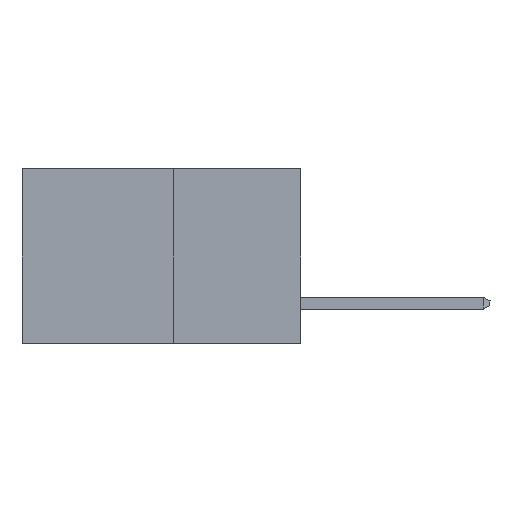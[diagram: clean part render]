
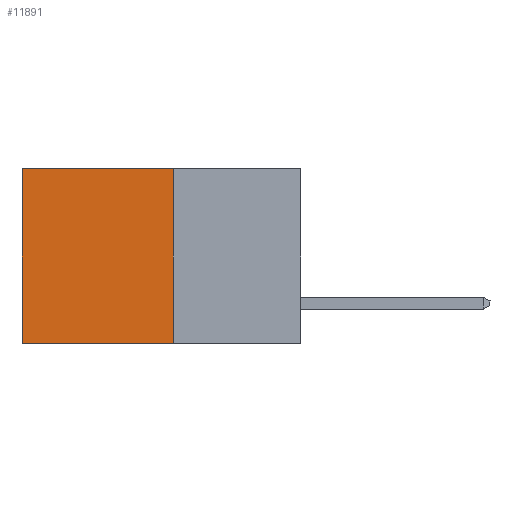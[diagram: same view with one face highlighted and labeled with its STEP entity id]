
A CAD part, left-side view. The second image highlights one B-rep face of the part: STEP entity #11891.
In plain terms, the highlighted planar face has unit normal (-1, 0, 0).
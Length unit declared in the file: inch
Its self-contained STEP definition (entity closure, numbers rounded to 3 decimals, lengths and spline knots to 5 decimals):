
#1458 = DIRECTION ( 'NONE',  ( 1., 0., 0. ) ) ;
#1577 = CARTESIAN_POINT ( 'NONE',  ( 0.277, 0.59, 0. ) ) ;
#1660 = VERTEX_POINT ( 'NONE', #1577 ) ;
#1937 = CARTESIAN_POINT ( 'NONE',  ( 0.277, 0.27, 0. ) ) ;
#2362 = DIRECTION ( 'NONE',  ( 0., 1., 0. ) ) ;
#2758 = LINE ( 'NONE', #12853, #5397 ) ;
#2946 = CARTESIAN_POINT ( 'NONE',  ( 0.277, 0.27, 0. ) ) ;
#2965 = DIRECTION ( 'NONE',  ( 0., 1., 0. ) ) ;
#3231 = VERTEX_POINT ( 'NONE', #8208 ) ;
#4039 = VERTEX_POINT ( 'NONE', #1937 ) ;
#4247 = ORIENTED_EDGE ( 'NONE', *, *, #6559, .T. ) ;
#4698 = EDGE_CURVE ( 'NONE', #4039, #1660, #4982, .T. ) ;
#4809 = VERTEX_POINT ( 'NONE', #12917 ) ;
#4841 = ORIENTED_EDGE ( 'NONE', *, *, #4698, .T. ) ;
#4982 = LINE ( 'NONE', #2946, #10055 ) ;
#5397 = VECTOR ( 'NONE', #9606, 39.37008 ) ;
#5882 = CARTESIAN_POINT ( 'NONE',  ( 0.277, 0.27, -0.37 ) ) ;
#6417 = CARTESIAN_POINT ( 'NONE',  ( 0.277, 0.27, -0.37 ) ) ;
#6559 = EDGE_CURVE ( 'NONE', #1660, #4809, #2758, .T. ) ;
#7026 = LINE ( 'NONE', #5882, #9393 ) ;
#7212 = ORIENTED_EDGE ( 'NONE', *, *, #7262, .F. ) ;
#7262 = EDGE_CURVE ( 'NONE', #4039, #3231, #12898, .T. ) ;
#7504 = ORIENTED_EDGE ( 'NONE', *, *, #12745, .F. ) ;
#7526 = CARTESIAN_POINT ( 'NONE',  ( 0.277, 0.27, -0.37 ) ) ;
#8208 = CARTESIAN_POINT ( 'NONE',  ( 0.277, 0.27, -0.37 ) ) ;
#8508 = DIRECTION ( 'NONE',  ( 0., 0., -1. ) ) ;
#9393 = VECTOR ( 'NONE', #2965, 39.37008 ) ;
#9435 = AXIS2_PLACEMENT_3D ( 'NONE', #7526, #1458, #8508 ) ;
#9606 = DIRECTION ( 'NONE',  ( 0., 0., -1. ) ) ;
#10055 = VECTOR ( 'NONE', #2362, 39.37008 ) ;
#10074 = DIRECTION ( 'NONE',  ( 0., 0., -1. ) ) ;
#10473 = VECTOR ( 'NONE', #10074, 39.37008 ) ;
#10513 = PLANE ( 'NONE',  #9435 ) ;
#11310 = FACE_OUTER_BOUND ( 'NONE', #12648, .T. ) ;
#11891 = ADVANCED_FACE ( 'NONE', ( #11310 ), #10513, .F. ) ;
#12648 = EDGE_LOOP ( 'NONE', ( #4247, #7504, #7212, #4841 ) ) ;
#12745 = EDGE_CURVE ( 'NONE', #3231, #4809, #7026, .T. ) ;
#12853 = CARTESIAN_POINT ( 'NONE',  ( 0.277, 0.59, -0.37 ) ) ;
#12898 = LINE ( 'NONE', #6417, #10473 ) ;
#12917 = CARTESIAN_POINT ( 'NONE',  ( 0.277, 0.59, -0.37 ) ) ;
